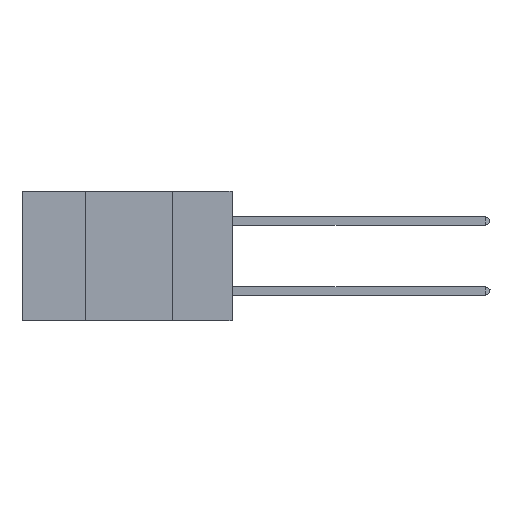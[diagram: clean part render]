
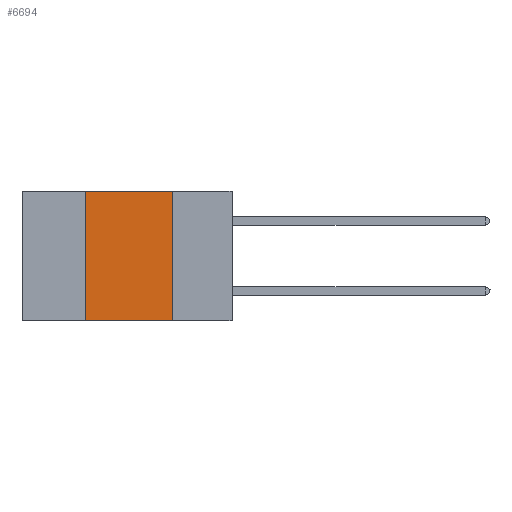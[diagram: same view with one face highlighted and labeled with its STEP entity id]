
A CAD part, left-side view. The second image highlights one B-rep face of the part: STEP entity #6694.
In plain terms, the highlighted planar face has unit normal (-1, 0, 0).
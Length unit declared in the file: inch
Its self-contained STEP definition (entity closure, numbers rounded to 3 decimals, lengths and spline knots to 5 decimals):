
#31 = VERTEX_POINT ( 'NONE', #12104 ) ;
#2033 = CARTESIAN_POINT ( 'NONE',  ( 0., 0.42, -0.37 ) ) ;
#2674 = DIRECTION ( 'NONE',  ( 0., 0., 1. ) ) ;
#2798 = DIRECTION ( 'NONE',  ( 0., -1., 0. ) ) ;
#2842 = ORIENTED_EDGE ( 'NONE', *, *, #33823, .F. ) ;
#5014 = VECTOR ( 'NONE', #31332, 39.37008 ) ;
#6296 = AXIS2_PLACEMENT_3D ( 'NONE', #7445, #18730, #18911 ) ;
#6694 = ADVANCED_FACE ( 'NONE', ( #12817 ), #32839, .F. ) ;
#7445 = CARTESIAN_POINT ( 'NONE',  ( 0., 0.6, 0. ) ) ;
#7960 = ORIENTED_EDGE ( 'NONE', *, *, #9203, .T. ) ;
#9203 = EDGE_CURVE ( 'NONE', #25542, #24189, #16688, .T. ) ;
#12104 = CARTESIAN_POINT ( 'NONE',  ( 0., 0.17, 0. ) ) ;
#12245 = LINE ( 'NONE', #29083, #5014 ) ;
#12817 = FACE_OUTER_BOUND ( 'NONE', #19307, .T. ) ;
#13967 = CARTESIAN_POINT ( 'NONE',  ( 0., 0.17, 0. ) ) ;
#16570 = DIRECTION ( 'NONE',  ( 0., 0., -1. ) ) ;
#16688 = LINE ( 'NONE', #22954, #34855 ) ;
#16746 = LINE ( 'NONE', #28037, #24021 ) ;
#17499 = EDGE_CURVE ( 'NONE', #29540, #31, #12245, .T. ) ;
#17503 = ORIENTED_EDGE ( 'NONE', *, *, #17499, .F. ) ;
#18341 = EDGE_CURVE ( 'NONE', #31, #24189, #33453, .T. ) ;
#18730 = DIRECTION ( 'NONE',  ( 1., 0., 0. ) ) ;
#18911 = DIRECTION ( 'NONE',  ( 0., 0., -1. ) ) ;
#19307 = EDGE_LOOP ( 'NONE', ( #25061, #17503, #2842, #7960 ) ) ;
#19802 = CARTESIAN_POINT ( 'NONE',  ( 0., 0.42, 0. ) ) ;
#22954 = CARTESIAN_POINT ( 'NONE',  ( 0., 0.6, -0.37 ) ) ;
#24021 = VECTOR ( 'NONE', #2674, 39.37008 ) ;
#24189 = VERTEX_POINT ( 'NONE', #31637 ) ;
#25061 = ORIENTED_EDGE ( 'NONE', *, *, #18341, .F. ) ;
#25542 = VERTEX_POINT ( 'NONE', #2033 ) ;
#25713 = VECTOR ( 'NONE', #16570, 39.37008 ) ;
#28037 = CARTESIAN_POINT ( 'NONE',  ( 0., 0.42, 0. ) ) ;
#29083 = CARTESIAN_POINT ( 'NONE',  ( 0., 0.6, 0. ) ) ;
#29540 = VERTEX_POINT ( 'NONE', #19802 ) ;
#31332 = DIRECTION ( 'NONE',  ( 0., -1., 0. ) ) ;
#31637 = CARTESIAN_POINT ( 'NONE',  ( 0., 0.17, -0.37 ) ) ;
#32839 = PLANE ( 'NONE',  #6296 ) ;
#33453 = LINE ( 'NONE', #13967, #25713 ) ;
#33823 = EDGE_CURVE ( 'NONE', #25542, #29540, #16746, .T. ) ;
#34855 = VECTOR ( 'NONE', #2798, 39.37008 ) ;
